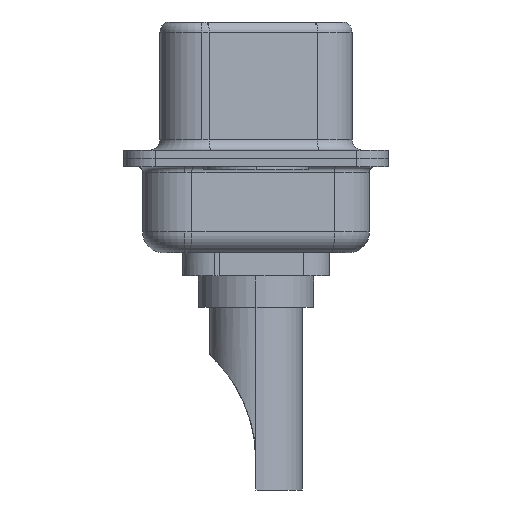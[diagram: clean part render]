
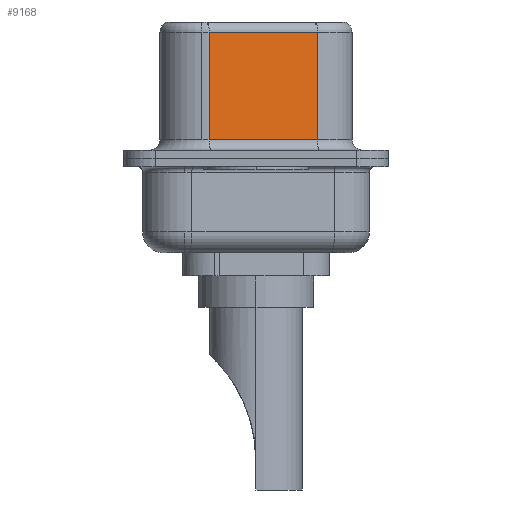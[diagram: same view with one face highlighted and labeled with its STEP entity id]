
A CAD part, left-side view. The second image highlights one B-rep face of the part: STEP entity #9168.
In plain terms, the highlighted planar face has unit normal (-0.985, -0.174, 0).
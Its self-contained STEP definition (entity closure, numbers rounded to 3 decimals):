
#160 = DIRECTION ( 'NONE',  ( 0., 0., -1. ) ) ;
#509 = EDGE_CURVE ( 'NONE', #963, #16309, #12384, .T. ) ;
#963 = VERTEX_POINT ( 'NONE', #12354 ) ;
#1004 = EDGE_CURVE ( 'NONE', #17548, #16044, #4864, .T. ) ;
#1303 = VECTOR ( 'NONE', #3046, 1000. ) ;
#2125 = LINE ( 'NONE', #4364, #1303 ) ;
#2228 = DIRECTION ( 'NONE',  ( 0.985, 0.174, 0. ) ) ;
#2555 = EDGE_CURVE ( 'NONE', #16044, #16309, #4589, .T. ) ;
#3046 = DIRECTION ( 'NONE',  ( -0.174, 0.985, 0. ) ) ;
#3168 = CARTESIAN_POINT ( 'NONE',  ( 3.67, 2.233, 6.02 ) ) ;
#3904 = CARTESIAN_POINT ( 'NONE',  ( 3.67, 2.233, 6.52 ) ) ;
#4265 = CARTESIAN_POINT ( 'NONE',  ( 4.58, -2.927, 6.52 ) ) ;
#4364 = CARTESIAN_POINT ( 'NONE',  ( 4.58, -2.927, 6.02 ) ) ;
#4589 = LINE ( 'NONE', #10629, #6710 ) ;
#4864 = LINE ( 'NONE', #3904, #6126 ) ;
#4914 = CARTESIAN_POINT ( 'NONE',  ( 4.58, -2.927, 6.52 ) ) ;
#6126 = VECTOR ( 'NONE', #13548, 1000. ) ;
#6350 = DIRECTION ( 'NONE',  ( -0.174, 0.985, 0. ) ) ;
#6710 = VECTOR ( 'NONE', #8207, 1000. ) ;
#7928 = FACE_OUTER_BOUND ( 'NONE', #15025, .T. ) ;
#8207 = DIRECTION ( 'NONE',  ( 0.174, -0.985, 0. ) ) ;
#8897 = CARTESIAN_POINT ( 'NONE',  ( 3.67, 2.233, 0.9 ) ) ;
#9168 = ADVANCED_FACE ( 'NONE', ( #7928 ), #13362, .F. ) ;
#9243 = ORIENTED_EDGE ( 'NONE', *, *, #1004, .T. ) ;
#9333 = EDGE_CURVE ( 'NONE', #963, #17548, #2125, .T. ) ;
#10629 = CARTESIAN_POINT ( 'NONE',  ( 4.58, -2.927, 0.9 ) ) ;
#12354 = CARTESIAN_POINT ( 'NONE',  ( 4.58, -2.927, 6.02 ) ) ;
#12384 = LINE ( 'NONE', #4265, #13235 ) ;
#13024 = AXIS2_PLACEMENT_3D ( 'NONE', #4914, #2228, #6350 ) ;
#13235 = VECTOR ( 'NONE', #160, 1000. ) ;
#13362 = PLANE ( 'NONE',  #13024 ) ;
#13548 = DIRECTION ( 'NONE',  ( 0., 0., -1. ) ) ;
#14374 = ORIENTED_EDGE ( 'NONE', *, *, #2555, .T. ) ;
#15025 = EDGE_LOOP ( 'NONE', ( #16127, #15457, #9243, #14374 ) ) ;
#15457 = ORIENTED_EDGE ( 'NONE', *, *, #9333, .T. ) ;
#16044 = VERTEX_POINT ( 'NONE', #8897 ) ;
#16127 = ORIENTED_EDGE ( 'NONE', *, *, #509, .F. ) ;
#16309 = VERTEX_POINT ( 'NONE', #16421 ) ;
#16421 = CARTESIAN_POINT ( 'NONE',  ( 4.58, -2.927, 0.9 ) ) ;
#17548 = VERTEX_POINT ( 'NONE', #3168 ) ;
